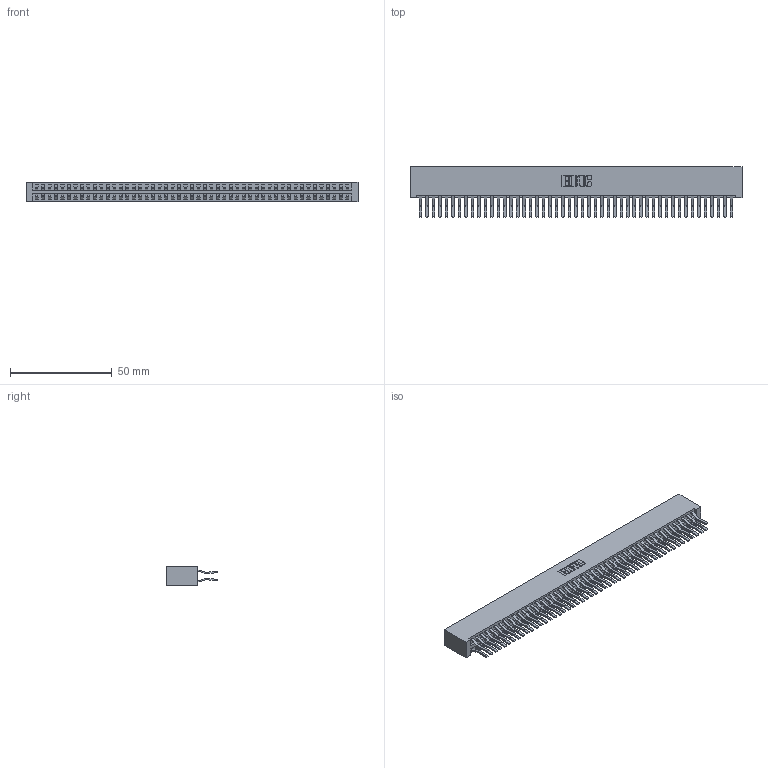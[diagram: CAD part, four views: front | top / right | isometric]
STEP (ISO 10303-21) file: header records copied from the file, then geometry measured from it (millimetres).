
FILE_DESCRIPTION (( 'STEP AP203' ), '1' );
FILE_NAME ('346-098-560-201.STEP', '2018-08-30T09:49:28', ( '' ), ( '' ), 'SwSTEP 2.0', 'SolidWorks 2016', '' );
FILE_SCHEMA (( 'CONFIG_CONTROL_DESIGN' ));
Length unit declared in the file: inch
Products named in the file (3): 346 Part_No Mounting Lugs; 345-292-001_560 Tail; 346-098-560-201
Assembly tree (99 placements, depth 2):
  346-098-560-201
    346 Part_No Mounting Lugs
    345-292-001_560 Tail  x98
Bounding box: 162.81 x 24.78 x 9.4 mm (x, y, z)
Volume: 17146.4 mm3; surface area: 25555.8 mm2
Topology: 99 solids, 99 shells, 5406 faces, 16083 edges, 10590 vertices
Faces by surface type: plane 3502, cylinder 1904
Entity records: 30847 total; most frequent: CARTESIAN_POINT 5072, ORIENTED_EDGE 5006, DIRECTION 4519, EDGE_CURVE 2503, LINE 2179, VECTOR 2179, VERTEX_POINT 1666, AXIS2_PLACEMENT_3D 1170
